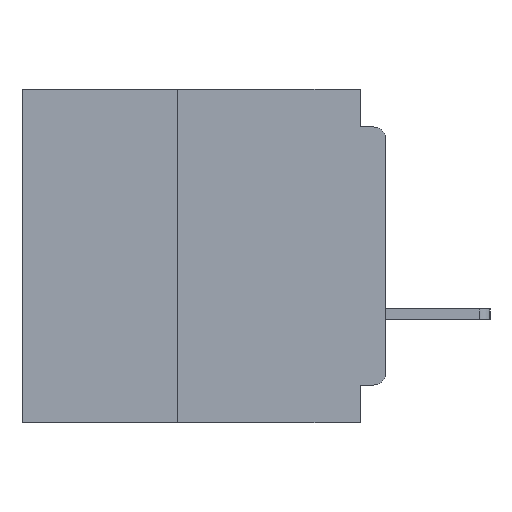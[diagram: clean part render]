
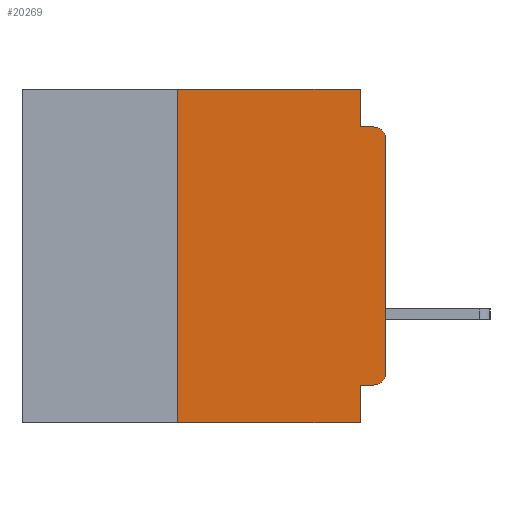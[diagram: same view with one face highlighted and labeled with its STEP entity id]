
A CAD part, left-side view. The second image highlights one B-rep face of the part: STEP entity #20269.
In plain terms, the highlighted planar face has unit normal (-1, 0, 0).
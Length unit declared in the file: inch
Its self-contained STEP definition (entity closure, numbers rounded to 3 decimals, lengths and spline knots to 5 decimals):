
#348 = VERTEX_POINT ( 'NONE', #32314 ) ;
#881 = DIRECTION ( 'NONE',  ( 0., 1., 0. ) ) ;
#1435 = CIRCLE ( 'NONE', #36668, 0.015 ) ;
#1862 = CARTESIAN_POINT ( 'NONE',  ( 0., 0.015, -0.34 ) ) ;
#2519 = VECTOR ( 'NONE', #35486, 39.37008 ) ;
#3014 = EDGE_CURVE ( 'NONE', #38783, #348, #42869, .T. ) ;
#3452 = VERTEX_POINT ( 'NONE', #23658 ) ;
#3519 = ORIENTED_EDGE ( 'NONE', *, *, #16977, .F. ) ;
#3661 = VECTOR ( 'NONE', #25854, 39.37008 ) ;
#4111 = DIRECTION ( 'NONE',  ( 0., -1., 0. ) ) ;
#4160 = VECTOR ( 'NONE', #10865, 39.37008 ) ;
#4495 = DIRECTION ( 'NONE',  ( -1., 0., 0. ) ) ;
#4946 = VECTOR ( 'NONE', #31275, 39.37008 ) ;
#4986 = CARTESIAN_POINT ( 'NONE',  ( 0., 0.437, 0. ) ) ;
#5101 = VERTEX_POINT ( 'NONE', #19343 ) ;
#5388 = DIRECTION ( 'NONE',  ( 0., 0., -1. ) ) ;
#5464 = EDGE_CURVE ( 'NONE', #13812, #3452, #39709, .T. ) ;
#5616 = CARTESIAN_POINT ( 'NONE',  ( 0., 0.015, -0.045 ) ) ;
#5768 = ORIENTED_EDGE ( 'NONE', *, *, #41715, .T. ) ;
#5940 = EDGE_LOOP ( 'NONE', ( #18028, #36373, #3519, #40155, #6832, #20853, #14878, #35949, #13858, #5768 ) ) ;
#6052 = LINE ( 'NONE', #34745, #4946 ) ;
#6293 = PLANE ( 'NONE',  #7228 ) ;
#6832 = ORIENTED_EDGE ( 'NONE', *, *, #3014, .F. ) ;
#7228 = AXIS2_PLACEMENT_3D ( 'NONE', #40850, #20298, #44268 ) ;
#7557 = CARTESIAN_POINT ( 'NONE',  ( 0., 0.031, -0.355 ) ) ;
#9149 = EDGE_CURVE ( 'NONE', #348, #16795, #6052, .T. ) ;
#10811 = CARTESIAN_POINT ( 'NONE',  ( 0., 0.437, -0.4 ) ) ;
#10865 = DIRECTION ( 'NONE',  ( 0., -1., 0. ) ) ;
#11215 = VERTEX_POINT ( 'NONE', #5616 ) ;
#11293 = CARTESIAN_POINT ( 'NONE',  ( 0., 0.25, 0. ) ) ;
#12364 = AXIS2_PLACEMENT_3D ( 'NONE', #1862, #26047, #5388 ) ;
#12513 = VERTEX_POINT ( 'NONE', #24595 ) ;
#13806 = CARTESIAN_POINT ( 'NONE',  ( 0., 0.031, -0.045 ) ) ;
#13812 = VERTEX_POINT ( 'NONE', #24631 ) ;
#13858 = ORIENTED_EDGE ( 'NONE', *, *, #36882, .F. ) ;
#14835 = CARTESIAN_POINT ( 'NONE',  ( 0., 0., -0.045 ) ) ;
#14878 = ORIENTED_EDGE ( 'NONE', *, *, #5464, .T. ) ;
#15535 = LINE ( 'NONE', #18157, #23673 ) ;
#16572 = DIRECTION ( 'NONE',  ( 0., 0., 1. ) ) ;
#16795 = VERTEX_POINT ( 'NONE', #13806 ) ;
#16977 = EDGE_CURVE ( 'NONE', #16795, #11215, #39206, .T. ) ;
#18028 = ORIENTED_EDGE ( 'NONE', *, *, #41302, .T. ) ;
#18157 = CARTESIAN_POINT ( 'NONE',  ( 0., 0., -0.355 ) ) ;
#19343 = CARTESIAN_POINT ( 'NONE',  ( 0., 0., -0.06 ) ) ;
#19910 = CARTESIAN_POINT ( 'NONE',  ( 0., 0., 0. ) ) ;
#20269 = ADVANCED_FACE ( 'NONE', ( #42666 ), #6293, .F. ) ;
#20298 = DIRECTION ( 'NONE',  ( 1., 0., 0. ) ) ;
#20853 = ORIENTED_EDGE ( 'NONE', *, *, #42287, .F. ) ;
#22404 = CARTESIAN_POINT ( 'NONE',  ( 0., 0.25, -0.4 ) ) ;
#23658 = CARTESIAN_POINT ( 'NONE',  ( 0., 0.031, -0.4 ) ) ;
#23673 = VECTOR ( 'NONE', #881, 39.37008 ) ;
#24461 = DIRECTION ( 'NONE',  ( 0., 0., -1. ) ) ;
#24595 = CARTESIAN_POINT ( 'NONE',  ( 0., 0., -0.34 ) ) ;
#24631 = CARTESIAN_POINT ( 'NONE',  ( 0., 0.25, -0.4 ) ) ;
#24681 = VECTOR ( 'NONE', #4111, 39.37008 ) ;
#25031 = EDGE_CURVE ( 'NONE', #40258, #3452, #37875, .T. ) ;
#25191 = CARTESIAN_POINT ( 'NONE',  ( 0., 0.015, -0.06 ) ) ;
#25854 = DIRECTION ( 'NONE',  ( 0., 0., 1. ) ) ;
#26047 = DIRECTION ( 'NONE',  ( -1., 0., 0. ) ) ;
#27467 = CIRCLE ( 'NONE', #12364, 0.015 ) ;
#27507 = VECTOR ( 'NONE', #16572, 39.37008 ) ;
#28159 = CARTESIAN_POINT ( 'NONE',  ( 0., 0.015, -0.355 ) ) ;
#28618 = DIRECTION ( 'NONE',  ( 0., 0., -1. ) ) ;
#30287 = VERTEX_POINT ( 'NONE', #28159 ) ;
#30892 = VECTOR ( 'NONE', #24461, 39.37008 ) ;
#31216 = CARTESIAN_POINT ( 'NONE',  ( 0., 0.031, -0.4 ) ) ;
#31275 = DIRECTION ( 'NONE',  ( 0., 0., -1. ) ) ;
#32314 = CARTESIAN_POINT ( 'NONE',  ( 0., 0.031, 0. ) ) ;
#34745 = CARTESIAN_POINT ( 'NONE',  ( 0., 0.031, 0. ) ) ;
#35486 = DIRECTION ( 'NONE',  ( 0., -1., 0. ) ) ;
#35949 = ORIENTED_EDGE ( 'NONE', *, *, #25031, .F. ) ;
#36373 = ORIENTED_EDGE ( 'NONE', *, *, #43008, .T. ) ;
#36641 = LINE ( 'NONE', #19910, #27507 ) ;
#36668 = AXIS2_PLACEMENT_3D ( 'NONE', #25191, #4495, #28618 ) ;
#36882 = EDGE_CURVE ( 'NONE', #30287, #40258, #15535, .T. ) ;
#37875 = LINE ( 'NONE', #31216, #30892 ) ;
#38783 = VERTEX_POINT ( 'NONE', #11293 ) ;
#39206 = LINE ( 'NONE', #14835, #2519 ) ;
#39709 = LINE ( 'NONE', #10811, #4160 ) ;
#40155 = ORIENTED_EDGE ( 'NONE', *, *, #9149, .F. ) ;
#40258 = VERTEX_POINT ( 'NONE', #7557 ) ;
#40282 = LINE ( 'NONE', #22404, #3661 ) ;
#40850 = CARTESIAN_POINT ( 'NONE',  ( 0., 0.437, 0. ) ) ;
#41302 = EDGE_CURVE ( 'NONE', #12513, #5101, #36641, .T. ) ;
#41715 = EDGE_CURVE ( 'NONE', #30287, #12513, #27467, .T. ) ;
#42287 = EDGE_CURVE ( 'NONE', #13812, #38783, #40282, .T. ) ;
#42666 = FACE_OUTER_BOUND ( 'NONE', #5940, .T. ) ;
#42869 = LINE ( 'NONE', #4986, #24681 ) ;
#43008 = EDGE_CURVE ( 'NONE', #5101, #11215, #1435, .T. ) ;
#44268 = DIRECTION ( 'NONE',  ( 0., 0., -1. ) ) ;
